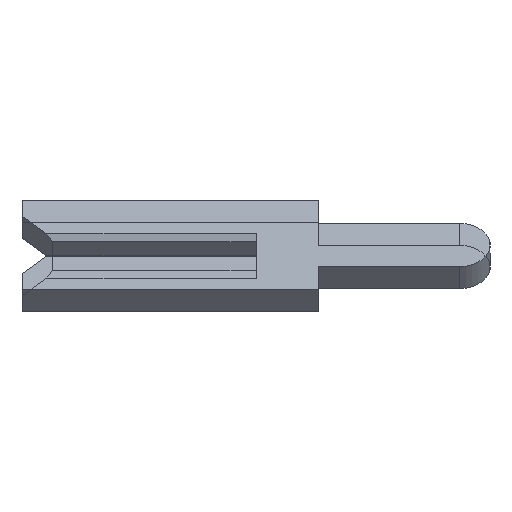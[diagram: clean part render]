
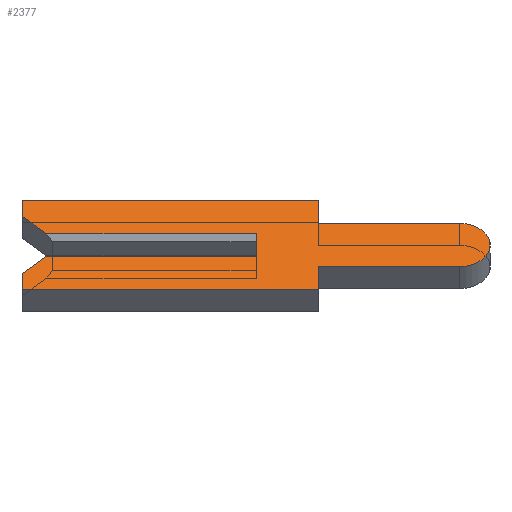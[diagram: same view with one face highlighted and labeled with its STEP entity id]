
A CAD part, left-side view. The second image highlights one B-rep face of the part: STEP entity #2377.
In plain terms, the highlighted face is planar.
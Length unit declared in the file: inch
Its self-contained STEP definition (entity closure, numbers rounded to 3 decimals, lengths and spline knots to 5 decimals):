
#1 = DIRECTION ( 'NONE',  ( 0., 0., 1. ) ) ;
#33 = VERTEX_POINT ( 'NONE', #2343 ) ;
#54 = CARTESIAN_POINT ( 'NONE',  ( -0.01, -0.04, -0.0195 ) ) ;
#88 = CARTESIAN_POINT ( 'NONE',  ( -0.01, -0.04, 0.04 ) ) ;
#128 = LINE ( 'NONE', #2219, #1784 ) ;
#131 = VECTOR ( 'NONE', #687, 39.37008 ) ;
#143 = DIRECTION ( 'NONE',  ( 0., -0.707, 0.707 ) ) ;
#155 = CARTESIAN_POINT ( 'NONE',  ( -0.01, -0.1305, 0. ) ) ;
#172 = CARTESIAN_POINT ( 'NONE',  ( -0.01, -0.04, 0.04 ) ) ;
#186 = VECTOR ( 'NONE', #1870, 39.37008 ) ;
#191 = ORIENTED_EDGE ( 'NONE', *, *, #209, .F. ) ;
#192 = VERTEX_POINT ( 'NONE', #2285 ) ;
#209 = EDGE_CURVE ( 'NONE', #192, #1266, #3138, .T. ) ;
#234 = CARTESIAN_POINT ( 'NONE',  ( -0.01, 0.15, 0.01 ) ) ;
#297 = LINE ( 'NONE', #3118, #3734 ) ;
#472 = DIRECTION ( 'NONE',  ( 1., 0., 0. ) ) ;
#504 = LINE ( 'NONE', #3938, #760 ) ;
#507 = LINE ( 'NONE', #3739, #3993 ) ;
#511 = LINE ( 'NONE', #54, #3893 ) ;
#515 = EDGE_CURVE ( 'NONE', #3593, #3486, #504, .T. ) ;
#601 = DIRECTION ( 'NONE',  ( 0., 0.707, 0.707 ) ) ;
#628 = CARTESIAN_POINT ( 'NONE',  ( -0.01, 0.1305, 0.0065 ) ) ;
#687 = DIRECTION ( 'NONE',  ( 0., 0., -1. ) ) ;
#711 = VECTOR ( 'NONE', #3192, 39.37008 ) ;
#721 = EDGE_CURVE ( 'NONE', #33, #3012, #511, .T. ) ;
#759 = DIRECTION ( 'NONE',  ( 0., 0., -1. ) ) ;
#760 = VECTOR ( 'NONE', #1, 39.37008 ) ;
#854 = CARTESIAN_POINT ( 'NONE',  ( -0.01, 0.15, -0.04 ) ) ;
#874 = DIRECTION ( 'NONE',  ( 0., 0., 1. ) ) ;
#904 = CARTESIAN_POINT ( 'NONE',  ( -0.01, 0.15, -0.04 ) ) ;
#905 = LINE ( 'NONE', #234, #186 ) ;
#964 = ORIENTED_EDGE ( 'NONE', *, *, #3149, .F. ) ;
#1013 = CARTESIAN_POINT ( 'NONE',  ( -0.01, 0.134, 0.01 ) ) ;
#1014 = VECTOR ( 'NONE', #1042, 39.37008 ) ;
#1016 = EDGE_CURVE ( 'NONE', #3486, #3361, #2466, .T. ) ;
#1032 = CARTESIAN_POINT ( 'NONE',  ( -0.01, -0.1305, 0.0195 ) ) ;
#1039 = VERTEX_POINT ( 'NONE', #1013 ) ;
#1042 = DIRECTION ( 'NONE',  ( 0., -1., 0. ) ) ;
#1081 = VERTEX_POINT ( 'NONE', #3045 ) ;
#1086 = ORIENTED_EDGE ( 'NONE', *, *, #2124, .F. ) ;
#1109 = DIRECTION ( 'NONE',  ( 1., 0., 0. ) ) ;
#1266 = VERTEX_POINT ( 'NONE', #1032 ) ;
#1337 = VECTOR ( 'NONE', #601, 39.37008 ) ;
#1349 = DIRECTION ( 'NONE',  ( 0., -1., 0. ) ) ;
#1389 = CARTESIAN_POINT ( 'NONE',  ( -0.01, 0.15, 0.04 ) ) ;
#1464 = EDGE_CURVE ( 'NONE', #3361, #192, #3533, .T. ) ;
#1486 = VECTOR ( 'NONE', #3251, 39.37008 ) ;
#1510 = CARTESIAN_POINT ( 'NONE',  ( -0.01, -0.04, -0.0195 ) ) ;
#1699 = VERTEX_POINT ( 'NONE', #1791 ) ;
#1700 = ORIENTED_EDGE ( 'NONE', *, *, #1464, .F. ) ;
#1758 = EDGE_CURVE ( 'NONE', #1699, #2074, #507, .T. ) ;
#1784 = VECTOR ( 'NONE', #874, 39.37008 ) ;
#1791 = CARTESIAN_POINT ( 'NONE',  ( -0.01, 0.15, -0.026 ) ) ;
#1810 = ORIENTED_EDGE ( 'NONE', *, *, #721, .F. ) ;
#1838 = CIRCLE ( 'NONE', #2567, 0.0195 ) ;
#1870 = DIRECTION ( 'NONE',  ( 0., -1., 0. ) ) ;
#1904 = CARTESIAN_POINT ( 'NONE',  ( -0.01, 0.15, 0.026 ) ) ;
#1944 = FACE_OUTER_BOUND ( 'NONE', #3806, .T. ) ;
#1955 = ORIENTED_EDGE ( 'NONE', *, *, #2069, .F. ) ;
#1974 = VERTEX_POINT ( 'NONE', #2126 ) ;
#2000 = LINE ( 'NONE', #628, #1337 ) ;
#2069 = EDGE_CURVE ( 'NONE', #1266, #33, #1838, .T. ) ;
#2074 = VERTEX_POINT ( 'NONE', #3390 ) ;
#2114 = PLANE ( 'NONE',  #2722 ) ;
#2124 = EDGE_CURVE ( 'NONE', #3012, #1081, #297, .T. ) ;
#2126 = CARTESIAN_POINT ( 'NONE',  ( -0.01, 0., -0.01 ) ) ;
#2130 = ORIENTED_EDGE ( 'NONE', *, *, #515, .F. ) ;
#2219 = CARTESIAN_POINT ( 'NONE',  ( -0.01, 0.15, -0.026 ) ) ;
#2252 = CARTESIAN_POINT ( 'NONE',  ( -0.01, 0.15, 0.04 ) ) ;
#2272 = VECTOR ( 'NONE', #1349, 39.37008 ) ;
#2285 = CARTESIAN_POINT ( 'NONE',  ( -0.01, -0.04, 0.0195 ) ) ;
#2343 = CARTESIAN_POINT ( 'NONE',  ( -0.01, -0.1305, -0.0195 ) ) ;
#2356 = DIRECTION ( 'NONE',  ( 0., 1., 0. ) ) ;
#2377 = ADVANCED_FACE ( 'NONE', ( #1944 ), #2114, .F. ) ;
#2420 = VECTOR ( 'NONE', #2907, 39.37008 ) ;
#2445 = CARTESIAN_POINT ( 'NONE',  ( -0.01, -0.1305, 0. ) ) ;
#2466 = LINE ( 'NONE', #1389, #1014 ) ;
#2514 = CARTESIAN_POINT ( 'NONE',  ( -0.01, 0., 0.01 ) ) ;
#2567 = AXIS2_PLACEMENT_3D ( 'NONE', #155, #1109, #3443 ) ;
#2587 = EDGE_CURVE ( 'NONE', #1974, #2920, #2673, .T. ) ;
#2673 = LINE ( 'NONE', #4113, #711 ) ;
#2678 = EDGE_CURVE ( 'NONE', #1039, #2920, #905, .T. ) ;
#2722 = AXIS2_PLACEMENT_3D ( 'NONE', #2445, #472, #759 ) ;
#2729 = VERTEX_POINT ( 'NONE', #854 ) ;
#2907 = DIRECTION ( 'NONE',  ( 0., -1., 0. ) ) ;
#2920 = VERTEX_POINT ( 'NONE', #2514 ) ;
#2939 = CARTESIAN_POINT ( 'NONE',  ( -0.01, -0.1305, -0.01 ) ) ;
#2974 = CARTESIAN_POINT ( 'NONE',  ( -0.01, -0.04, 0.0195 ) ) ;
#3012 = VERTEX_POINT ( 'NONE', #1510 ) ;
#3045 = CARTESIAN_POINT ( 'NONE',  ( -0.01, -0.04, -0.04 ) ) ;
#3118 = CARTESIAN_POINT ( 'NONE',  ( -0.01, -0.04, -0.04 ) ) ;
#3129 = LINE ( 'NONE', #904, #1486 ) ;
#3138 = LINE ( 'NONE', #2974, #2272 ) ;
#3149 = EDGE_CURVE ( 'NONE', #2729, #1699, #128, .T. ) ;
#3192 = DIRECTION ( 'NONE',  ( 0., 0., 1. ) ) ;
#3251 = DIRECTION ( 'NONE',  ( 0., 1., 0. ) ) ;
#3361 = VERTEX_POINT ( 'NONE', #172 ) ;
#3385 = ORIENTED_EDGE ( 'NONE', *, *, #2587, .F. ) ;
#3390 = CARTESIAN_POINT ( 'NONE',  ( -0.01, 0.134, -0.01 ) ) ;
#3409 = DIRECTION ( 'NONE',  ( 0., 0., -1. ) ) ;
#3443 = DIRECTION ( 'NONE',  ( 0., 0., -1. ) ) ;
#3486 = VERTEX_POINT ( 'NONE', #2252 ) ;
#3533 = LINE ( 'NONE', #88, #131 ) ;
#3593 = VERTEX_POINT ( 'NONE', #1904 ) ;
#3604 = EDGE_CURVE ( 'NONE', #1081, #2729, #3129, .T. ) ;
#3639 = ORIENTED_EDGE ( 'NONE', *, *, #2678, .T. ) ;
#3671 = ORIENTED_EDGE ( 'NONE', *, *, #3793, .F. ) ;
#3734 = VECTOR ( 'NONE', #3409, 39.37008 ) ;
#3736 = ORIENTED_EDGE ( 'NONE', *, *, #1758, .F. ) ;
#3739 = CARTESIAN_POINT ( 'NONE',  ( -0.01, 0.1305, -0.0065 ) ) ;
#3793 = EDGE_CURVE ( 'NONE', #2074, #1974, #4089, .T. ) ;
#3806 = EDGE_LOOP ( 'NONE', ( #3639, #3385, #3671, #3736, #964, #4100, #1086, #1810, #1955, #191, #1700, #4143, #2130, #3946 ) ) ;
#3870 = EDGE_CURVE ( 'NONE', #1039, #3593, #2000, .T. ) ;
#3893 = VECTOR ( 'NONE', #2356, 39.37008 ) ;
#3938 = CARTESIAN_POINT ( 'NONE',  ( -0.01, 0.15, 0.026 ) ) ;
#3946 = ORIENTED_EDGE ( 'NONE', *, *, #3870, .F. ) ;
#3993 = VECTOR ( 'NONE', #143, 39.37008 ) ;
#4089 = LINE ( 'NONE', #2939, #2420 ) ;
#4100 = ORIENTED_EDGE ( 'NONE', *, *, #3604, .F. ) ;
#4113 = CARTESIAN_POINT ( 'NONE',  ( -0.01, 0., 0.0065 ) ) ;
#4143 = ORIENTED_EDGE ( 'NONE', *, *, #1016, .F. ) ;
